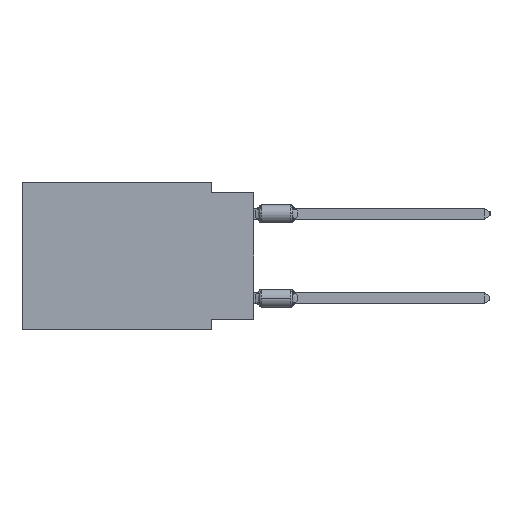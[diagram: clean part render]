
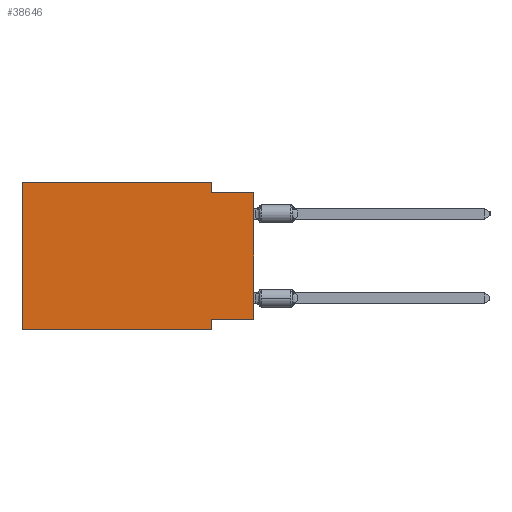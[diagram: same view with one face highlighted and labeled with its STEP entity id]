
A CAD part, left-side view. The second image highlights one B-rep face of the part: STEP entity #38646.
In plain terms, the highlighted planar face has unit normal (-1, 0, 0).
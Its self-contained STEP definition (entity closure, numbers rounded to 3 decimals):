
#622 = LINE ( 'NONE', #8043, #7315 ) ;
#1409 = EDGE_CURVE ( 'NONE', #5912, #30268, #622, .T. ) ;
#1950 = EDGE_CURVE ( 'NONE', #9400, #13231, #13703, .T. ) ;
#2110 = CARTESIAN_POINT ( 'NONE',  ( 0., 2.54, -8.89 ) ) ;
#2325 = VECTOR ( 'NONE', #45310, 1000. ) ;
#2566 = CARTESIAN_POINT ( 'NONE',  ( 0., 0., 0. ) ) ;
#2893 = EDGE_CURVE ( 'NONE', #17460, #12331, #15147, .T. ) ;
#3094 = EDGE_CURVE ( 'NONE', #13231, #12331, #9746, .T. ) ;
#3673 = ORIENTED_EDGE ( 'NONE', *, *, #3094, .F. ) ;
#4685 = DIRECTION ( 'NONE',  ( 0., -1., 0. ) ) ;
#4746 = DIRECTION ( 'NONE',  ( 0., -1., 0. ) ) ;
#4954 = ORIENTED_EDGE ( 'NONE', *, *, #19671, .F. ) ;
#5912 = VERTEX_POINT ( 'NONE', #37611 ) ;
#6798 = EDGE_CURVE ( 'NONE', #9400, #27241, #31613, .T. ) ;
#7315 = VECTOR ( 'NONE', #22216, 1000. ) ;
#7862 = DIRECTION ( 'NONE',  ( 1., 0., 0. ) ) ;
#8043 = CARTESIAN_POINT ( 'NONE',  ( 0., 2.54, 0. ) ) ;
#8090 = DIRECTION ( 'NONE',  ( 0., 0., -1. ) ) ;
#8386 = CARTESIAN_POINT ( 'NONE',  ( 0., 13.97, 0. ) ) ;
#8770 = VECTOR ( 'NONE', #4685, 1000. ) ;
#9151 = CARTESIAN_POINT ( 'NONE',  ( 0., 0., -8.255 ) ) ;
#9400 = VERTEX_POINT ( 'NONE', #28883 ) ;
#9746 = LINE ( 'NONE', #2110, #41453 ) ;
#11062 = ORIENTED_EDGE ( 'NONE', *, *, #43442, .F. ) ;
#11993 = VECTOR ( 'NONE', #25749, 1000. ) ;
#12158 = VECTOR ( 'NONE', #29549, 1000. ) ;
#12331 = VERTEX_POINT ( 'NONE', #43800 ) ;
#12976 = CARTESIAN_POINT ( 'NONE',  ( 0., 2.54, -8.255 ) ) ;
#13231 = VERTEX_POINT ( 'NONE', #12976 ) ;
#13703 = LINE ( 'NONE', #9151, #42217 ) ;
#15147 = LINE ( 'NONE', #32816, #8770 ) ;
#15509 = LINE ( 'NONE', #26655, #11993 ) ;
#17460 = VERTEX_POINT ( 'NONE', #21323 ) ;
#19671 = EDGE_CURVE ( 'NONE', #21999, #5912, #15509, .T. ) ;
#19924 = ORIENTED_EDGE ( 'NONE', *, *, #1950, .F. ) ;
#21323 = CARTESIAN_POINT ( 'NONE',  ( 0., 13.97, -8.89 ) ) ;
#21365 = DIRECTION ( 'NONE',  ( 0., 1., 0. ) ) ;
#21999 = VERTEX_POINT ( 'NONE', #35142 ) ;
#22151 = EDGE_CURVE ( 'NONE', #17460, #21999, #32572, .T. ) ;
#22216 = DIRECTION ( 'NONE',  ( 0., 0., -1. ) ) ;
#22773 = VECTOR ( 'NONE', #4746, 1000. ) ;
#25593 = EDGE_LOOP ( 'NONE', ( #36448, #11062, #31543, #4954, #31233, #35195, #3673, #19924 ) ) ;
#25726 = AXIS2_PLACEMENT_3D ( 'NONE', #29014, #7862, #8090 ) ;
#25749 = DIRECTION ( 'NONE',  ( 0., -1., 0. ) ) ;
#26575 = LINE ( 'NONE', #26798, #22773 ) ;
#26655 = CARTESIAN_POINT ( 'NONE',  ( 0., 13.97, 0. ) ) ;
#26798 = CARTESIAN_POINT ( 'NONE',  ( 0., 0., -0.635 ) ) ;
#27241 = VERTEX_POINT ( 'NONE', #31404 ) ;
#28883 = CARTESIAN_POINT ( 'NONE',  ( 0., 0., -8.255 ) ) ;
#29014 = CARTESIAN_POINT ( 'NONE',  ( 0., 13.97, 0. ) ) ;
#29549 = DIRECTION ( 'NONE',  ( 0., 0., 1. ) ) ;
#30268 = VERTEX_POINT ( 'NONE', #33345 ) ;
#31233 = ORIENTED_EDGE ( 'NONE', *, *, #22151, .F. ) ;
#31404 = CARTESIAN_POINT ( 'NONE',  ( 0., 0., -0.635 ) ) ;
#31543 = ORIENTED_EDGE ( 'NONE', *, *, #1409, .F. ) ;
#31613 = LINE ( 'NONE', #2566, #2325 ) ;
#32572 = LINE ( 'NONE', #8386, #12158 ) ;
#32816 = CARTESIAN_POINT ( 'NONE',  ( 0., 13.97, -8.89 ) ) ;
#33345 = CARTESIAN_POINT ( 'NONE',  ( 0., 2.54, -0.635 ) ) ;
#35142 = CARTESIAN_POINT ( 'NONE',  ( 0., 13.97, 0. ) ) ;
#35195 = ORIENTED_EDGE ( 'NONE', *, *, #2893, .T. ) ;
#36448 = ORIENTED_EDGE ( 'NONE', *, *, #6798, .T. ) ;
#37450 = DIRECTION ( 'NONE',  ( 0., 0., -1. ) ) ;
#37611 = CARTESIAN_POINT ( 'NONE',  ( 0., 2.54, 0. ) ) ;
#38646 = ADVANCED_FACE ( 'NONE', ( #39015 ), #39472, .F. ) ;
#39015 = FACE_OUTER_BOUND ( 'NONE', #25593, .T. ) ;
#39472 = PLANE ( 'NONE',  #25726 ) ;
#41453 = VECTOR ( 'NONE', #37450, 1000. ) ;
#42217 = VECTOR ( 'NONE', #21365, 1000. ) ;
#43442 = EDGE_CURVE ( 'NONE', #30268, #27241, #26575, .T. ) ;
#43800 = CARTESIAN_POINT ( 'NONE',  ( 0., 2.54, -8.89 ) ) ;
#45310 = DIRECTION ( 'NONE',  ( 0., 0., 1. ) ) ;
